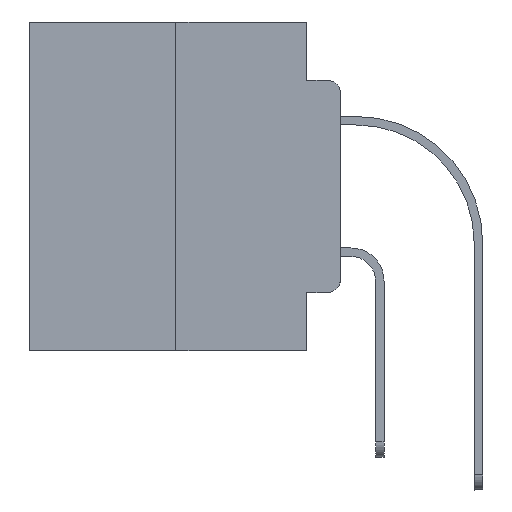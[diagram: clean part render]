
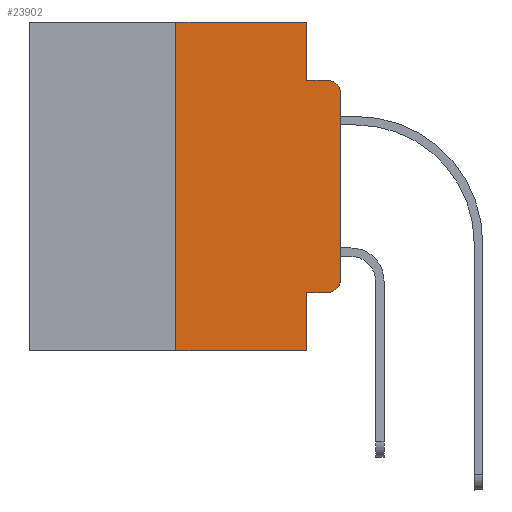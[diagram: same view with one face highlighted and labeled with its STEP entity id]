
A CAD part, left-side view. The second image highlights one B-rep face of the part: STEP entity #23902.
In plain terms, the highlighted planar face has unit normal (-1, 0, 0).
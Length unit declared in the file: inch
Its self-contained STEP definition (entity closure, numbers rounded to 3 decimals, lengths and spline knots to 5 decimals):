
#255 = ORIENTED_EDGE ( 'NONE', *, *, #21368, .F. ) ;
#645 = DIRECTION ( 'NONE',  ( 0., 0., 1. ) ) ;
#917 = CARTESIAN_POINT ( 'NONE',  ( 0., 0.051, -0.4115 ) ) ;
#1454 = CARTESIAN_POINT ( 'NONE',  ( 0., 0.051, -0.5 ) ) ;
#1547 = DIRECTION ( 'NONE',  ( 0., -1., 0. ) ) ;
#1809 = CARTESIAN_POINT ( 'NONE',  ( 0., 0.02, -0.3915 ) ) ;
#2164 = DIRECTION ( 'NONE',  ( 0., -1., 0. ) ) ;
#2354 = EDGE_CURVE ( 'NONE', #23089, #10682, #15122, .T. ) ;
#2483 = CARTESIAN_POINT ( 'NONE',  ( 0., 0.473, 0. ) ) ;
#2718 = VERTEX_POINT ( 'NONE', #5401 ) ;
#3225 = DIRECTION ( 'NONE',  ( 0., 0., -1. ) ) ;
#3404 = CARTESIAN_POINT ( 'NONE',  ( 0., 0., 0. ) ) ;
#4656 = DIRECTION ( 'NONE',  ( 1., 0., 0. ) ) ;
#5049 = LINE ( 'NONE', #26694, #9562 ) ;
#5229 = DIRECTION ( 'NONE',  ( -1., 0., 0. ) ) ;
#5258 = ORIENTED_EDGE ( 'NONE', *, *, #2354, .F. ) ;
#5374 = VERTEX_POINT ( 'NONE', #1454 ) ;
#5401 = CARTESIAN_POINT ( 'NONE',  ( 0., 0.051, -0.0885 ) ) ;
#6471 = CARTESIAN_POINT ( 'NONE',  ( 0., 0., -0.3915 ) ) ;
#7039 = ORIENTED_EDGE ( 'NONE', *, *, #16939, .T. ) ;
#7264 = CIRCLE ( 'NONE', #27082, 0.02 ) ;
#7842 = LINE ( 'NONE', #16664, #8807 ) ;
#8078 = ORIENTED_EDGE ( 'NONE', *, *, #21799, .F. ) ;
#8143 = DIRECTION ( 'NONE',  ( -1., 0., 0. ) ) ;
#8320 = DIRECTION ( 'NONE',  ( 0., 0., 1. ) ) ;
#8515 = LINE ( 'NONE', #17334, #28445 ) ;
#8807 = VECTOR ( 'NONE', #18663, 39.37008 ) ;
#9235 = DIRECTION ( 'NONE',  ( 0., -1., 0. ) ) ;
#9313 = CARTESIAN_POINT ( 'NONE',  ( 0., 0.25, 0. ) ) ;
#9405 = FACE_OUTER_BOUND ( 'NONE', #25020, .T. ) ;
#9442 = VECTOR ( 'NONE', #645, 39.37008 ) ;
#9562 = VECTOR ( 'NONE', #9235, 39.37008 ) ;
#10133 = ORIENTED_EDGE ( 'NONE', *, *, #19748, .T. ) ;
#10312 = EDGE_CURVE ( 'NONE', #14760, #23089, #12841, .T. ) ;
#10372 = AXIS2_PLACEMENT_3D ( 'NONE', #14184, #5229, #3225 ) ;
#10620 = DIRECTION ( 'NONE',  ( 0., 0., -1. ) ) ;
#10682 = VERTEX_POINT ( 'NONE', #19252 ) ;
#10912 = EDGE_CURVE ( 'NONE', #18692, #13730, #21450, .T. ) ;
#10981 = VERTEX_POINT ( 'NONE', #917 ) ;
#12841 = LINE ( 'NONE', #9313, #9442 ) ;
#13328 = PLANE ( 'NONE',  #13798 ) ;
#13659 = CARTESIAN_POINT ( 'NONE',  ( 0., 0.051, 0. ) ) ;
#13730 = VERTEX_POINT ( 'NONE', #17738 ) ;
#13798 = AXIS2_PLACEMENT_3D ( 'NONE', #2483, #4656, #18225 ) ;
#14034 = ORIENTED_EDGE ( 'NONE', *, *, #10912, .T. ) ;
#14164 = CARTESIAN_POINT ( 'NONE',  ( 0., 0., -0.1085 ) ) ;
#14184 = CARTESIAN_POINT ( 'NONE',  ( 0., 0.02, -0.1085 ) ) ;
#14760 = VERTEX_POINT ( 'NONE', #25678 ) ;
#14967 = CARTESIAN_POINT ( 'NONE',  ( 0., 0.473, 0. ) ) ;
#15122 = LINE ( 'NONE', #14967, #18827 ) ;
#15507 = ORIENTED_EDGE ( 'NONE', *, *, #10312, .F. ) ;
#15559 = DIRECTION ( 'NONE',  ( 0., 0., -1. ) ) ;
#16557 = CARTESIAN_POINT ( 'NONE',  ( 0., 0.25, 0. ) ) ;
#16664 = CARTESIAN_POINT ( 'NONE',  ( 0., 0.051, -0.4115 ) ) ;
#16939 = EDGE_CURVE ( 'NONE', #26188, #21730, #7264, .T. ) ;
#17334 = CARTESIAN_POINT ( 'NONE',  ( 0., 0.473, -0.5 ) ) ;
#17738 = CARTESIAN_POINT ( 'NONE',  ( 0., 0.02, -0.0885 ) ) ;
#17886 = ORIENTED_EDGE ( 'NONE', *, *, #22713, .F. ) ;
#18017 = LINE ( 'NONE', #13659, #23440 ) ;
#18225 = DIRECTION ( 'NONE',  ( 0., 0., -1. ) ) ;
#18663 = DIRECTION ( 'NONE',  ( 0., -1., 0. ) ) ;
#18692 = VERTEX_POINT ( 'NONE', #14164 ) ;
#18827 = VECTOR ( 'NONE', #1547, 39.37008 ) ;
#18894 = LINE ( 'NONE', #27818, #22035 ) ;
#19252 = CARTESIAN_POINT ( 'NONE',  ( 0., 0.051, 0. ) ) ;
#19748 = EDGE_CURVE ( 'NONE', #10981, #26188, #7842, .T. ) ;
#20247 = ORIENTED_EDGE ( 'NONE', *, *, #24507, .T. ) ;
#21368 = EDGE_CURVE ( 'NONE', #2718, #13730, #5049, .T. ) ;
#21450 = CIRCLE ( 'NONE', #10372, 0.02 ) ;
#21730 = VERTEX_POINT ( 'NONE', #6471 ) ;
#21799 = EDGE_CURVE ( 'NONE', #10682, #2718, #18017, .T. ) ;
#22035 = VECTOR ( 'NONE', #27686, 39.37008 ) ;
#22402 = EDGE_CURVE ( 'NONE', #14760, #5374, #8515, .T. ) ;
#22713 = EDGE_CURVE ( 'NONE', #10981, #5374, #18894, .T. ) ;
#22745 = CARTESIAN_POINT ( 'NONE',  ( 0., 0.02, -0.4115 ) ) ;
#23089 = VERTEX_POINT ( 'NONE', #16557 ) ;
#23189 = LINE ( 'NONE', #3404, #25807 ) ;
#23440 = VECTOR ( 'NONE', #15559, 39.37008 ) ;
#23902 = ADVANCED_FACE ( 'NONE', ( #9405 ), #13328, .F. ) ;
#24507 = EDGE_CURVE ( 'NONE', #21730, #18692, #23189, .T. ) ;
#25020 = EDGE_LOOP ( 'NONE', ( #20247, #14034, #255, #8078, #5258, #15507, #25376, #17886, #10133, #7039 ) ) ;
#25376 = ORIENTED_EDGE ( 'NONE', *, *, #22402, .T. ) ;
#25678 = CARTESIAN_POINT ( 'NONE',  ( 0., 0.25, -0.5 ) ) ;
#25807 = VECTOR ( 'NONE', #8320, 39.37008 ) ;
#26188 = VERTEX_POINT ( 'NONE', #22745 ) ;
#26694 = CARTESIAN_POINT ( 'NONE',  ( 0., 0.051, -0.0885 ) ) ;
#27082 = AXIS2_PLACEMENT_3D ( 'NONE', #1809, #8143, #10620 ) ;
#27686 = DIRECTION ( 'NONE',  ( 0., 0., -1. ) ) ;
#27818 = CARTESIAN_POINT ( 'NONE',  ( 0., 0.051, 0. ) ) ;
#28445 = VECTOR ( 'NONE', #2164, 39.37008 ) ;
